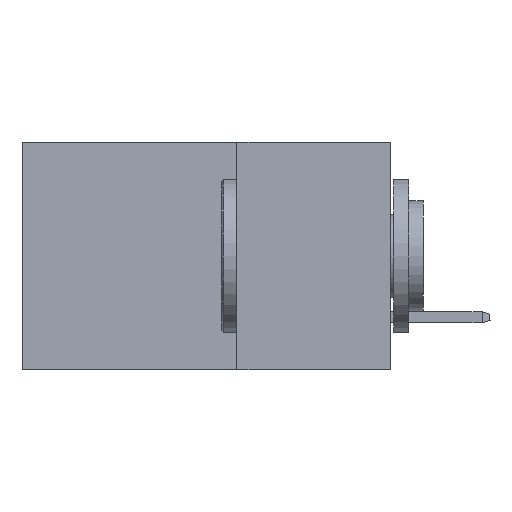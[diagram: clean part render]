
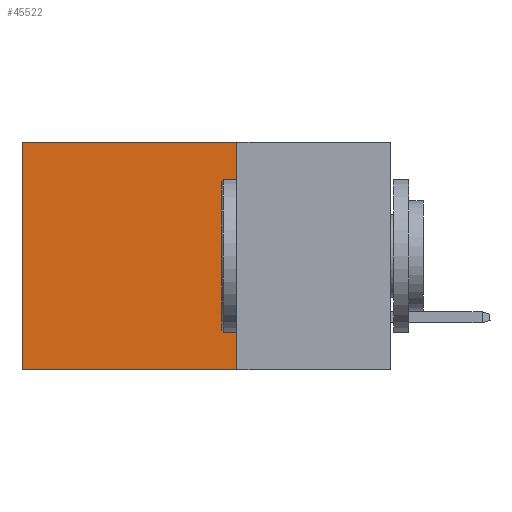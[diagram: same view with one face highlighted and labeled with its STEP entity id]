
A CAD part, left-side view. The second image highlights one B-rep face of the part: STEP entity #45522.
In plain terms, the highlighted planar face has unit normal (-1, 0, 0).
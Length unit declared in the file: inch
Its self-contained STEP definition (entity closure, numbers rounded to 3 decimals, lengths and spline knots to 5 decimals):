
#1119 = DIRECTION ( 'NONE',  ( 1., 0., 0. ) ) ;
#2432 = ORIENTED_EDGE ( 'NONE', *, *, #35666, .F. ) ;
#4334 = LINE ( 'NONE', #6473, #45804 ) ;
#4962 = AXIS2_PLACEMENT_3D ( 'NONE', #8649, #1119, #12895 ) ;
#5115 = VERTEX_POINT ( 'NONE', #38701 ) ;
#6450 = VECTOR ( 'NONE', #33451, 39.37008 ) ;
#6473 = CARTESIAN_POINT ( 'NONE',  ( 0.2875, 0.25, 0. ) ) ;
#7549 = CARTESIAN_POINT ( 'NONE',  ( 0.2875, 0.6, -0.37 ) ) ;
#8649 = CARTESIAN_POINT ( 'NONE',  ( 0.2875, 0.25, 0. ) ) ;
#9136 = VECTOR ( 'NONE', #46688, 39.37008 ) ;
#10739 = EDGE_CURVE ( 'NONE', #21732, #40221, #28936, .T. ) ;
#12450 = CARTESIAN_POINT ( 'NONE',  ( 0.2875, 0.25, -0.37 ) ) ;
#12895 = DIRECTION ( 'NONE',  ( 0., 0., -1. ) ) ;
#13578 = CARTESIAN_POINT ( 'NONE',  ( 0.2875, 0.6, 0. ) ) ;
#14079 = DIRECTION ( 'NONE',  ( 0., 1., 0. ) ) ;
#16262 = CARTESIAN_POINT ( 'NONE',  ( 0.2875, 0.6, 0. ) ) ;
#18478 = VERTEX_POINT ( 'NONE', #34535 ) ;
#20999 = FACE_OUTER_BOUND ( 'NONE', #47018, .T. ) ;
#21400 = CARTESIAN_POINT ( 'NONE',  ( 0.2875, 0.25, 0. ) ) ;
#21732 = VERTEX_POINT ( 'NONE', #16262 ) ;
#24227 = EDGE_CURVE ( 'NONE', #5115, #18478, #4334, .T. ) ;
#25577 = ORIENTED_EDGE ( 'NONE', *, *, #10739, .T. ) ;
#27190 = LINE ( 'NONE', #21400, #27255 ) ;
#27255 = VECTOR ( 'NONE', #14079, 39.37008 ) ;
#27407 = LINE ( 'NONE', #12450, #6450 ) ;
#27667 = PLANE ( 'NONE',  #4962 ) ;
#28936 = LINE ( 'NONE', #13578, #9136 ) ;
#32110 = ORIENTED_EDGE ( 'NONE', *, *, #24227, .F. ) ;
#32539 = DIRECTION ( 'NONE',  ( 0., 0., -1. ) ) ;
#33451 = DIRECTION ( 'NONE',  ( 0., 1., 0. ) ) ;
#34535 = CARTESIAN_POINT ( 'NONE',  ( 0.2875, 0.25, -0.37 ) ) ;
#35666 = EDGE_CURVE ( 'NONE', #18478, #40221, #27407, .T. ) ;
#38701 = CARTESIAN_POINT ( 'NONE',  ( 0.2875, 0.25, 0. ) ) ;
#40221 = VERTEX_POINT ( 'NONE', #7549 ) ;
#43161 = EDGE_CURVE ( 'NONE', #5115, #21732, #27190, .T. ) ;
#45522 = ADVANCED_FACE ( 'NONE', ( #20999 ), #27667, .F. ) ;
#45804 = VECTOR ( 'NONE', #32539, 39.37008 ) ;
#46688 = DIRECTION ( 'NONE',  ( 0., 0., -1. ) ) ;
#47018 = EDGE_LOOP ( 'NONE', ( #25577, #2432, #32110, #47462 ) ) ;
#47462 = ORIENTED_EDGE ( 'NONE', *, *, #43161, .T. ) ;
